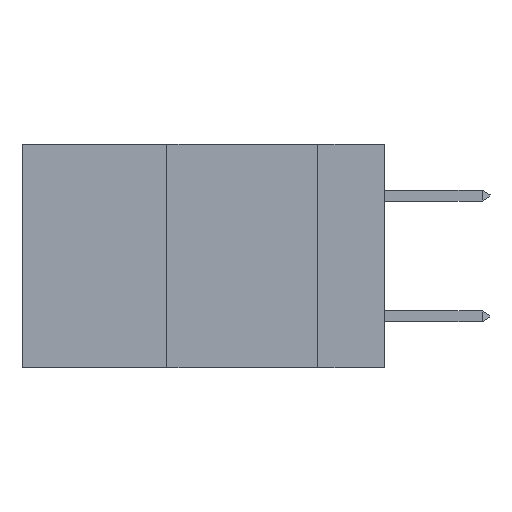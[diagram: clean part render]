
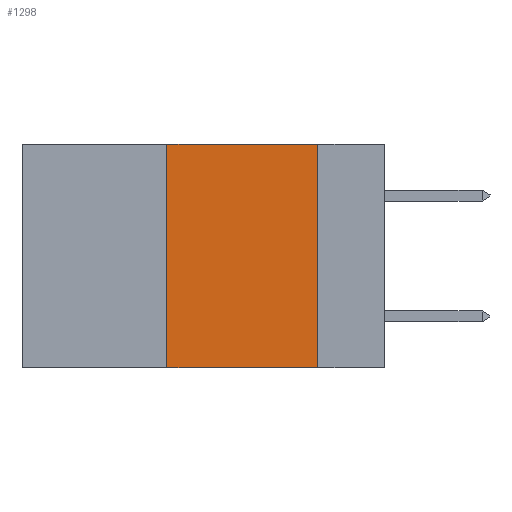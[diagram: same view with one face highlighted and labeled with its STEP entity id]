
A CAD part, left-side view. The second image highlights one B-rep face of the part: STEP entity #1298.
In plain terms, the highlighted planar face has unit normal (-1, 0, 0).
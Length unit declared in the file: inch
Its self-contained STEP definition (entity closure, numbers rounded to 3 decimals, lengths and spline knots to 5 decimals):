
#1298 = ADVANCED_FACE ( 'NONE', ( #17369 ), #7559, .F. ) ;
#2914 = LINE ( 'NONE', #30931, #3772 ) ;
#3216 = CARTESIAN_POINT ( 'NONE',  ( 0., 0.6, -0.37 ) ) ;
#3772 = VECTOR ( 'NONE', #7926, 39.37008 ) ;
#6945 = CARTESIAN_POINT ( 'NONE',  ( 0., 0.6, 0. ) ) ;
#7181 = DIRECTION ( 'NONE',  ( 0., 0., -1. ) ) ;
#7395 = VECTOR ( 'NONE', #35455, 39.37008 ) ;
#7465 = EDGE_LOOP ( 'NONE', ( #13526, #16878, #7767, #17707 ) ) ;
#7559 = PLANE ( 'NONE',  #24596 ) ;
#7767 = ORIENTED_EDGE ( 'NONE', *, *, #26376, .F. ) ;
#7926 = DIRECTION ( 'NONE',  ( 0., 0., -1. ) ) ;
#8786 = LINE ( 'NONE', #6945, #11522 ) ;
#9492 = VERTEX_POINT ( 'NONE', #21130 ) ;
#11235 = LINE ( 'NONE', #21322, #30735 ) ;
#11522 = VECTOR ( 'NONE', #15594, 39.37008 ) ;
#13526 = ORIENTED_EDGE ( 'NONE', *, *, #18988, .F. ) ;
#15594 = DIRECTION ( 'NONE',  ( 0., -1., 0. ) ) ;
#16878 = ORIENTED_EDGE ( 'NONE', *, *, #29269, .F. ) ;
#17369 = FACE_OUTER_BOUND ( 'NONE', #7465, .T. ) ;
#17682 = CARTESIAN_POINT ( 'NONE',  ( 0., 0.11, 0. ) ) ;
#17706 = VERTEX_POINT ( 'NONE', #33656 ) ;
#17707 = ORIENTED_EDGE ( 'NONE', *, *, #19328, .T. ) ;
#18988 = EDGE_CURVE ( 'NONE', #22268, #9492, #2914, .T. ) ;
#19328 = EDGE_CURVE ( 'NONE', #17706, #9492, #29230, .T. ) ;
#21130 = CARTESIAN_POINT ( 'NONE',  ( 0., 0.11, -0.37 ) ) ;
#21322 = CARTESIAN_POINT ( 'NONE',  ( 0., 0.36, 0. ) ) ;
#21495 = CARTESIAN_POINT ( 'NONE',  ( 0., 0.6, 0. ) ) ;
#22268 = VERTEX_POINT ( 'NONE', #17682 ) ;
#24596 = AXIS2_PLACEMENT_3D ( 'NONE', #21495, #27868, #7181 ) ;
#26376 = EDGE_CURVE ( 'NONE', #17706, #29157, #11235, .T. ) ;
#27868 = DIRECTION ( 'NONE',  ( 1., 0., 0. ) ) ;
#29157 = VERTEX_POINT ( 'NONE', #35396 ) ;
#29230 = LINE ( 'NONE', #3216, #7395 ) ;
#29269 = EDGE_CURVE ( 'NONE', #29157, #22268, #8786, .T. ) ;
#30135 = DIRECTION ( 'NONE',  ( 0., 0., 1. ) ) ;
#30735 = VECTOR ( 'NONE', #30135, 39.37008 ) ;
#30931 = CARTESIAN_POINT ( 'NONE',  ( 0., 0.11, 0. ) ) ;
#33656 = CARTESIAN_POINT ( 'NONE',  ( 0., 0.36, -0.37 ) ) ;
#35396 = CARTESIAN_POINT ( 'NONE',  ( 0., 0.36, 0. ) ) ;
#35455 = DIRECTION ( 'NONE',  ( 0., -1., 0. ) ) ;
